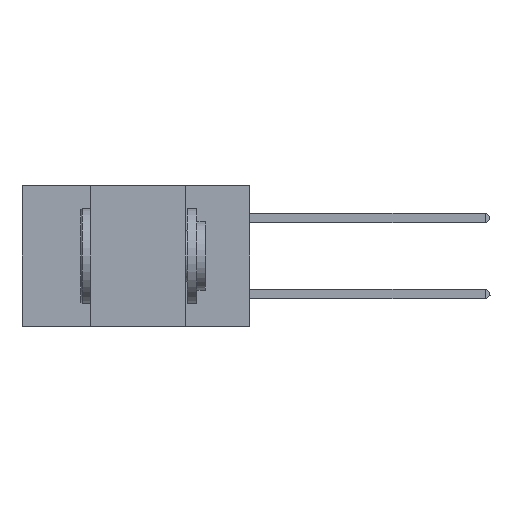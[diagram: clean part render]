
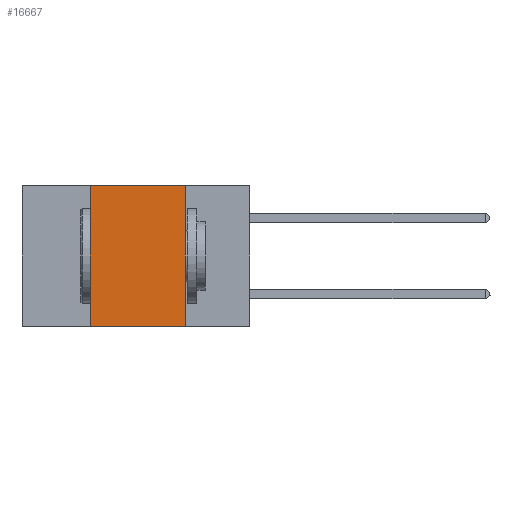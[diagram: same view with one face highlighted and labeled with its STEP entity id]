
A CAD part, left-side view. The second image highlights one B-rep face of the part: STEP entity #16667.
In plain terms, the highlighted planar face has unit normal (-1, 0, 0).
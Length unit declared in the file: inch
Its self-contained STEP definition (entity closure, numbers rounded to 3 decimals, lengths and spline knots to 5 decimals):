
#852 = CARTESIAN_POINT ( 'NONE',  ( 0., 0.42, 0. ) ) ;
#965 = EDGE_CURVE ( 'NONE', #10426, #3194, #13646, .T. ) ;
#1629 = VERTEX_POINT ( 'NONE', #27263 ) ;
#1631 = EDGE_CURVE ( 'NONE', #1629, #18220, #32779, .T. ) ;
#3194 = VERTEX_POINT ( 'NONE', #13826 ) ;
#3643 = VECTOR ( 'NONE', #22260, 39.37008 ) ;
#4825 = AXIS2_PLACEMENT_3D ( 'NONE', #20937, #31119, #26952 ) ;
#6009 = CARTESIAN_POINT ( 'NONE',  ( 0., 0.6, -0.37 ) ) ;
#6949 = EDGE_CURVE ( 'NONE', #10426, #18220, #20597, .T. ) ;
#10426 = VERTEX_POINT ( 'NONE', #25942 ) ;
#11278 = CARTESIAN_POINT ( 'NONE',  ( 0., 0.6, 0. ) ) ;
#12393 = CARTESIAN_POINT ( 'NONE',  ( 0., 0.17, -0.37 ) ) ;
#13646 = LINE ( 'NONE', #852, #3643 ) ;
#13826 = CARTESIAN_POINT ( 'NONE',  ( 0., 0.42, 0. ) ) ;
#14193 = CARTESIAN_POINT ( 'NONE',  ( 0., 0.17, 0. ) ) ;
#14677 = ORIENTED_EDGE ( 'NONE', *, *, #18719, .F. ) ;
#15805 = VECTOR ( 'NONE', #24103, 39.37008 ) ;
#16667 = ADVANCED_FACE ( 'NONE', ( #25378 ), #28533, .F. ) ;
#17762 = EDGE_LOOP ( 'NONE', ( #19388, #14677, #18252, #26909 ) ) ;
#18220 = VERTEX_POINT ( 'NONE', #12393 ) ;
#18252 = ORIENTED_EDGE ( 'NONE', *, *, #965, .F. ) ;
#18719 = EDGE_CURVE ( 'NONE', #3194, #1629, #22383, .T. ) ;
#19388 = ORIENTED_EDGE ( 'NONE', *, *, #1631, .F. ) ;
#20597 = LINE ( 'NONE', #6009, #15805 ) ;
#20937 = CARTESIAN_POINT ( 'NONE',  ( 0., 0.6, 0. ) ) ;
#21986 = DIRECTION ( 'NONE',  ( 0., 0., -1. ) ) ;
#22260 = DIRECTION ( 'NONE',  ( 0., 0., 1. ) ) ;
#22383 = LINE ( 'NONE', #11278, #27597 ) ;
#24103 = DIRECTION ( 'NONE',  ( 0., -1., 0. ) ) ;
#25378 = FACE_OUTER_BOUND ( 'NONE', #17762, .T. ) ;
#25942 = CARTESIAN_POINT ( 'NONE',  ( 0., 0.42, -0.37 ) ) ;
#26906 = DIRECTION ( 'NONE',  ( 0., -1., 0. ) ) ;
#26909 = ORIENTED_EDGE ( 'NONE', *, *, #6949, .T. ) ;
#26952 = DIRECTION ( 'NONE',  ( 0., 0., -1. ) ) ;
#27263 = CARTESIAN_POINT ( 'NONE',  ( 0., 0.17, 0. ) ) ;
#27597 = VECTOR ( 'NONE', #26906, 39.37008 ) ;
#28533 = PLANE ( 'NONE',  #4825 ) ;
#29563 = VECTOR ( 'NONE', #21986, 39.37008 ) ;
#31119 = DIRECTION ( 'NONE',  ( 1., 0., 0. ) ) ;
#32779 = LINE ( 'NONE', #14193, #29563 ) ;
